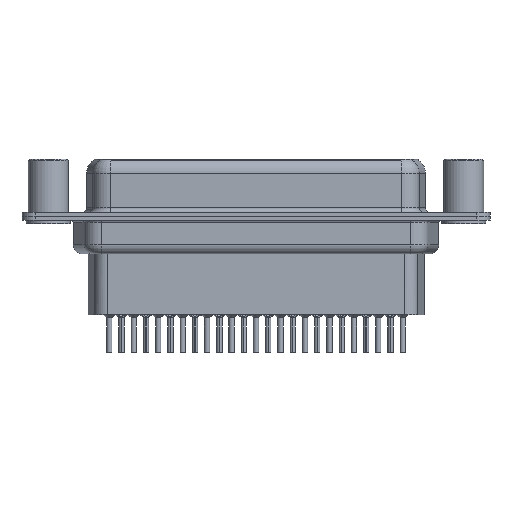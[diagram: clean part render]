
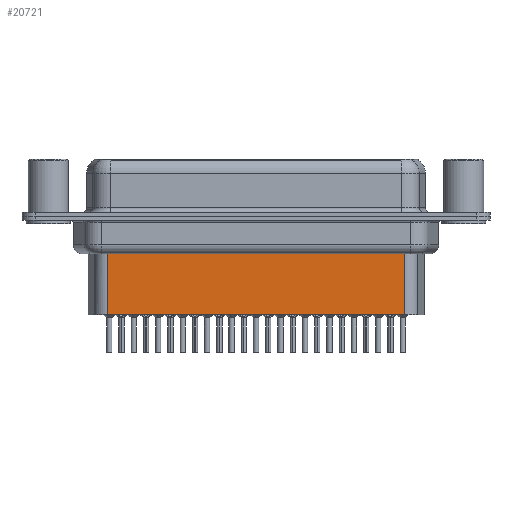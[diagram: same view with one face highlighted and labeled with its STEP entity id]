
A CAD part, front view. The second image highlights one B-rep face of the part: STEP entity #20721.
In plain terms, the highlighted planar face has unit normal (0, -1, 0).
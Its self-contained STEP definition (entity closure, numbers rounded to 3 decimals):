
#33 = CARTESIAN_POINT ( 'NONE',  ( 40.344, -3.5, -4.097 ) ) ;
#1814 = PLANE ( 'NONE',  #26576 ) ;
#2375 = EDGE_CURVE ( 'NONE', #10887, #21678, #23558, .T. ) ;
#3481 = VECTOR ( 'NONE', #4261, 1000. ) ;
#3755 = DIRECTION ( 'NONE',  ( 0., 0., -1. ) ) ;
#4254 = CARTESIAN_POINT ( 'NONE',  ( 6.706, -3.5, -4.097 ) ) ;
#4261 = DIRECTION ( 'NONE',  ( -1., 0., 0. ) ) ;
#5778 = CARTESIAN_POINT ( 'NONE',  ( 6.706, -3.5, -3.1 ) ) ;
#6301 = CARTESIAN_POINT ( 'NONE',  ( 40.344, -3.5, -11.15 ) ) ;
#6762 = VECTOR ( 'NONE', #17279, 1000. ) ;
#8261 = FACE_OUTER_BOUND ( 'NONE', #9933, .T. ) ;
#8549 = DIRECTION ( 'NONE',  ( 1., 0., 0. ) ) ;
#9933 = EDGE_LOOP ( 'NONE', ( #24943, #25472, #24317, #19639 ) ) ;
#10412 = EDGE_CURVE ( 'NONE', #22425, #21678, #25710, .T. ) ;
#10887 = VERTEX_POINT ( 'NONE', #6301 ) ;
#10996 = LINE ( 'NONE', #14898, #3481 ) ;
#11059 = LINE ( 'NONE', #14963, #12543 ) ;
#12543 = VECTOR ( 'NONE', #3755, 1000. ) ;
#12807 = CARTESIAN_POINT ( 'NONE',  ( 6.706, -3.5, -11.15 ) ) ;
#12962 = VERTEX_POINT ( 'NONE', #33 ) ;
#14637 = DIRECTION ( 'NONE',  ( 0., 0., -1. ) ) ;
#14898 = CARTESIAN_POINT ( 'NONE',  ( 6.459, -3.5, -4.097 ) ) ;
#14963 = CARTESIAN_POINT ( 'NONE',  ( 40.344, -3.5, -3.1 ) ) ;
#17279 = DIRECTION ( 'NONE',  ( -1., 0., 0. ) ) ;
#19577 = CARTESIAN_POINT ( 'NONE',  ( 6.706, -3.5, -3.1 ) ) ;
#19639 = ORIENTED_EDGE ( 'NONE', *, *, #2375, .F. ) ;
#20503 = CARTESIAN_POINT ( 'NONE',  ( 6.706, -3.5, -11.15 ) ) ;
#20721 = ADVANCED_FACE ( 'NONE', ( #8261 ), #1814, .T. ) ;
#21678 = VERTEX_POINT ( 'NONE', #20503 ) ;
#22425 = VERTEX_POINT ( 'NONE', #4254 ) ;
#23558 = LINE ( 'NONE', #12807, #6762 ) ;
#23657 = EDGE_CURVE ( 'NONE', #12962, #22425, #10996, .T. ) ;
#24146 = VECTOR ( 'NONE', #14637, 1000. ) ;
#24317 = ORIENTED_EDGE ( 'NONE', *, *, #10412, .T. ) ;
#24943 = ORIENTED_EDGE ( 'NONE', *, *, #25505, .F. ) ;
#25472 = ORIENTED_EDGE ( 'NONE', *, *, #23657, .T. ) ;
#25505 = EDGE_CURVE ( 'NONE', #12962, #10887, #11059, .T. ) ;
#25710 = LINE ( 'NONE', #5778, #24146 ) ;
#26576 = AXIS2_PLACEMENT_3D ( 'NONE', #19577, #28459, #8549 ) ;
#28459 = DIRECTION ( 'NONE',  ( 0., -1., 0. ) ) ;
